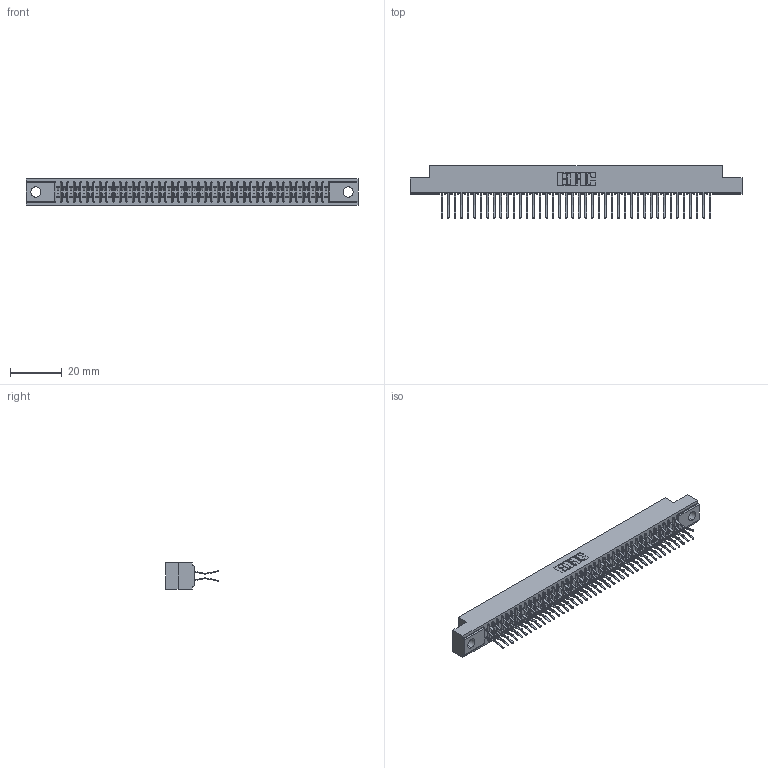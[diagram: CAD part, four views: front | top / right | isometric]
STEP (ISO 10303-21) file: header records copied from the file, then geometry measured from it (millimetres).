
FILE_DESCRIPTION (( 'STEP AP203' ), '1' );
FILE_NAME ('341-084-560-204.STEP', '2018-08-07T22:52:14', ( '' ), ( '' ), 'SwSTEP 2.0', 'SolidWorks 2016', '' );
FILE_SCHEMA (( 'CONFIG_CONTROL_DESIGN' ));
Length unit declared in the file: inch
Products named in the file (3): 341 Part_.156 (3.96) Dia Mounting Holes; 341-292-001_341-292-160; 341-084-560-204
Assembly tree (85 placements, depth 2):
  341-084-560-204
    341 Part_.156 (3.96) Dia Mounting Holes
    341-292-001_341-292-160  x84
Bounding box: 128.91 x 20.37 x 10.16 mm (x, y, z)
Volume: 9496.4 mm3; surface area: 17365.5 mm2
Topology: 85 solids, 85 shells, 6010 faces, 17446 edges, 11318 vertices
Faces by surface type: plane 3442, cylinder 2400, sphere 86, torus 82
Entity records: 51387 total; most frequent: CARTESIAN_POINT 8548, ORIENTED_EDGE 8492, DIRECTION 8292, EDGE_CURVE 4246, VECTOR 3432, LINE 3432, VERTEX_POINT 2686, AXIS2_PLACEMENT_3D 2430
